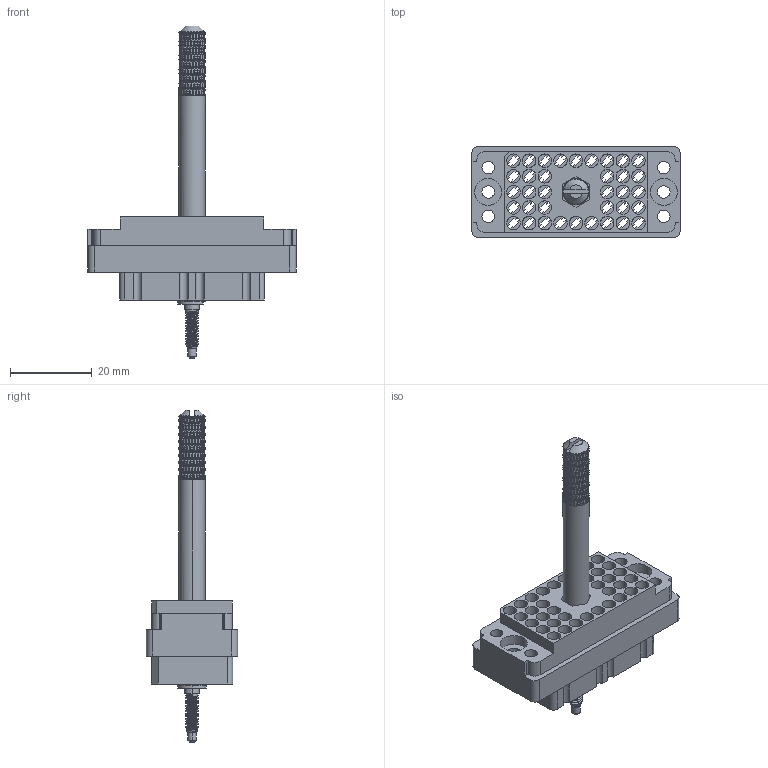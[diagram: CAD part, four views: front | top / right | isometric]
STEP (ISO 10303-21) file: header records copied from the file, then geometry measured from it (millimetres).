
FILE_DESCRIPTION (( 'STEP AP203' ), '1' );
FILE_NAME ('519-036-000-405.STEP', '2020-09-09T19:44:59', ( '' ), ( '' ), 'SwSTEP 2.0', 'SolidWorks 2020', '' );
FILE_SCHEMA (( 'CONFIG_CONTROL_DESIGN' ));
Length unit declared in the file: inch
Products named in the file (7): 519-036-000-405; 516-251-035-100; 516-253-035-100; 519 Receptacle Insulator_036; 516-250-038-111; 516-253-138-107; Actuating Screw Assy 038-056
Assembly tree (7 placements, depth 3):
  519-036-000-405
    519 Receptacle Insulator_036
    Actuating Screw Assy 038-056
      516-251-035-100
      516-253-035-100  x2
      516-253-138-107
      516-250-038-111
Bounding box: 50.8 x 22.25 x 81.03 mm (x, y, z)
Volume: 13134.1 mm3; surface area: 16065.8 mm2
Topology: 6 solids, 6 shells, 2247 faces, 5483 edges, 3268 vertices
Faces by surface type: bspline 1006, plane 687, cylinder 534, cone 20
Entity records: 95269 total; most frequent: CARTESIAN_POINT 53146, ORIENTED_EDGE 10942, DIRECTION 6100, EDGE_CURVE 5471, VERTEX_POINT 3260, EDGE_LOOP 2351, FACE_OUTER_BOUND 2241, ADVANCED_FACE 2241
